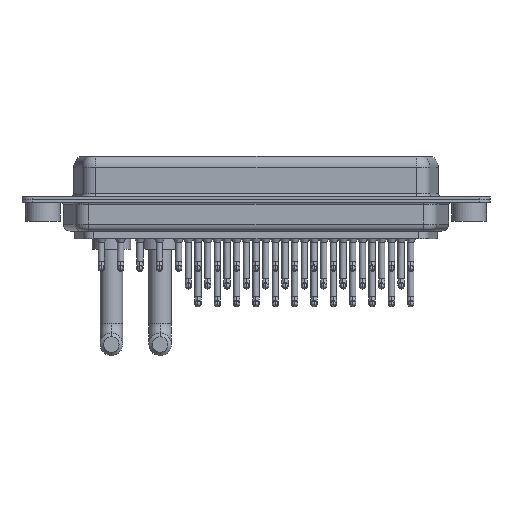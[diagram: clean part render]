
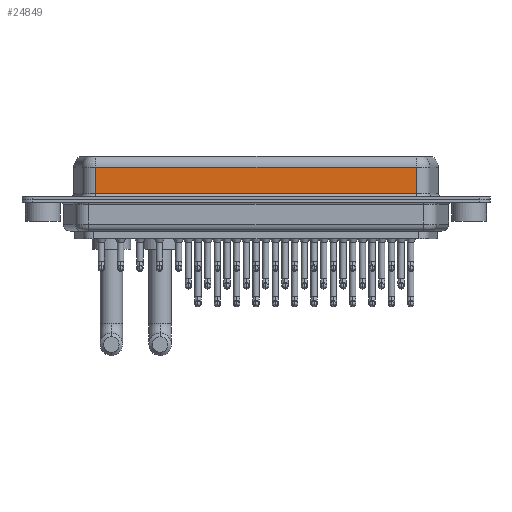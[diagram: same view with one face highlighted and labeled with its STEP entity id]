
A CAD part, front view. The second image highlights one B-rep face of the part: STEP entity #24849.
In plain terms, the highlighted planar face has unit normal (0, -1, 0).
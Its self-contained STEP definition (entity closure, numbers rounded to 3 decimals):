
#2834 = CARTESIAN_POINT ( 'NONE',  ( 53.41, -5.375, 4.65 ) ) ;
#3173 = CARTESIAN_POINT ( 'NONE',  ( 53.41, -5.375, 6.4 ) ) ;
#3397 = CARTESIAN_POINT ( 'NONE',  ( 53.41, -5.375, 0.9 ) ) ;
#4322 = ORIENTED_EDGE ( 'NONE', *, *, #4634, .T. ) ;
#4634 = EDGE_CURVE ( 'NONE', #11091, #31566, #5662, .T. ) ;
#4963 = ORIENTED_EDGE ( 'NONE', *, *, #19825, .T. ) ;
#5173 = CARTESIAN_POINT ( 'NONE',  ( 7.59, -5.375, 6.4 ) ) ;
#5662 = LINE ( 'NONE', #5173, #28551 ) ;
#6121 = DIRECTION ( 'NONE',  ( 0., 1., 0. ) ) ;
#6196 = LINE ( 'NONE', #6848, #6231 ) ;
#6231 = VECTOR ( 'NONE', #16576, 1000. ) ;
#6386 = VERTEX_POINT ( 'NONE', #2834 ) ;
#6606 = CARTESIAN_POINT ( 'NONE',  ( 53.41, -5.375, 6.4 ) ) ;
#6848 = CARTESIAN_POINT ( 'NONE',  ( 53.41, -5.375, 4.65 ) ) ;
#10837 = EDGE_CURVE ( 'NONE', #31566, #27859, #30604, .T. ) ;
#11091 = VERTEX_POINT ( 'NONE', #24489 ) ;
#11379 = EDGE_LOOP ( 'NONE', ( #31668, #4963, #4322, #26740 ) ) ;
#11563 = FACE_OUTER_BOUND ( 'NONE', #11379, .T. ) ;
#13239 = DIRECTION ( 'NONE',  ( 0., 0., -1. ) ) ;
#15717 = LINE ( 'NONE', #3173, #28509 ) ;
#15782 = DIRECTION ( 'NONE',  ( 1., 0., 0. ) ) ;
#15928 = AXIS2_PLACEMENT_3D ( 'NONE', #6606, #6121, #16665 ) ;
#16576 = DIRECTION ( 'NONE',  ( -1., 0., 0. ) ) ;
#16665 = DIRECTION ( 'NONE',  ( 0., 0., 1. ) ) ;
#18024 = DIRECTION ( 'NONE',  ( 0., 0., -1. ) ) ;
#19505 = CARTESIAN_POINT ( 'NONE',  ( 7.59, -5.375, 0.9 ) ) ;
#19825 = EDGE_CURVE ( 'NONE', #6386, #11091, #6196, .T. ) ;
#21448 = VECTOR ( 'NONE', #15782, 1000. ) ;
#24489 = CARTESIAN_POINT ( 'NONE',  ( 7.59, -5.375, 4.65 ) ) ;
#24849 = ADVANCED_FACE ( 'NONE', ( #11563 ), #28680, .F. ) ;
#26740 = ORIENTED_EDGE ( 'NONE', *, *, #10837, .T. ) ;
#27859 = VERTEX_POINT ( 'NONE', #32445 ) ;
#28509 = VECTOR ( 'NONE', #13239, 1000. ) ;
#28551 = VECTOR ( 'NONE', #18024, 1000. ) ;
#28680 = PLANE ( 'NONE',  #15928 ) ;
#30339 = EDGE_CURVE ( 'NONE', #6386, #27859, #15717, .T. ) ;
#30604 = LINE ( 'NONE', #3397, #21448 ) ;
#31566 = VERTEX_POINT ( 'NONE', #19505 ) ;
#31668 = ORIENTED_EDGE ( 'NONE', *, *, #30339, .F. ) ;
#32445 = CARTESIAN_POINT ( 'NONE',  ( 53.41, -5.375, 0.9 ) ) ;
